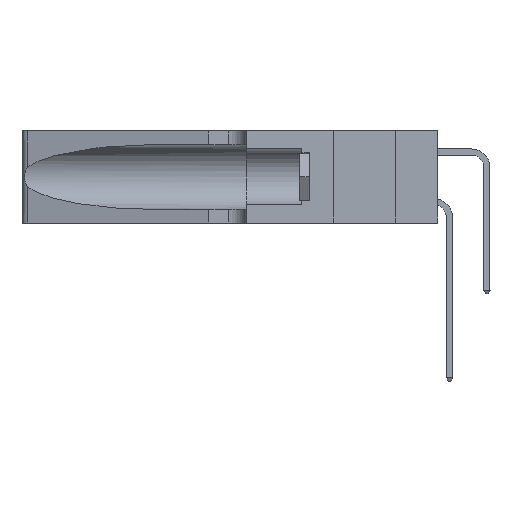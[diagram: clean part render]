
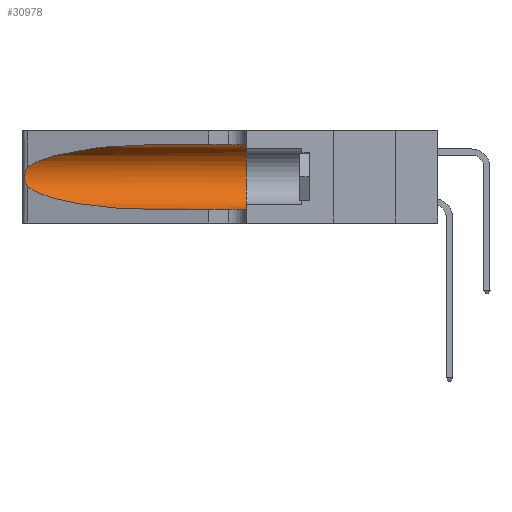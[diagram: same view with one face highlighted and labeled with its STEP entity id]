
A CAD part, left-side view. The second image highlights one B-rep face of the part: STEP entity #30978.
In plain terms, the highlighted cylindrical face has radius 3.308 mm (diameter 6.617 mm), a partial arc.
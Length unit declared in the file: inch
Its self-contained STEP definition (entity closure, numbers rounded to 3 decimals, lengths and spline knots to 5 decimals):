
#34 = CARTESIAN_POINT ( 'NONE',  ( 0.25856, 1.23593, 0.16098 ) ) ;
#484 = CARTESIAN_POINT ( 'NONE',  ( 0.1305, 0.35, 0.185 ) ) ;
#785 = CARTESIAN_POINT ( 'NONE',  ( 0.25487, 1.22718, 0.14631 ) ) ;
#837 = VERTEX_POINT ( 'NONE', #17722 ) ;
#2016 = EDGE_CURVE ( 'NONE', #837, #20874, #7929, .T. ) ;
#2540 = CARTESIAN_POINT ( 'NONE',  ( 0.25487, 1.22718, 0.22369 ) ) ;
#2912 = CARTESIAN_POINT ( 'NONE',  ( 0.25789, 1.23486, 0.15765 ) ) ;
#3282 = CARTESIAN_POINT ( 'NONE',  ( 0.1305, 1.61858, 0.185 ) ) ;
#3753 = CIRCLE ( 'NONE', #21391, 0.13025 ) ;
#3768 = CARTESIAN_POINT ( 'NONE',  ( 0.1305, 0.35, 0.31525 ) ) ;
#4000 = VERTEX_POINT ( 'NONE', #28427 ) ;
#4106 = EDGE_CURVE ( 'NONE', #36669, #4000, #4164, .T. ) ;
#4164 = LINE ( 'NONE', #28540, #14040 ) ;
#5214 = B_SPLINE_CURVE_WITH_KNOTS ( 'NONE', 3,
 ( #2540, #19873, #22757, #31066, #11403, #31175, #34190, #17014, #14859, #34, #2912, #28343, #11272, #25711 ),
 .UNSPECIFIED., .F., .F.,
 ( 4, 2, 2, 2, 2, 2, 4 ),
 ( 0., 0.00027, 0.00053, 0.00107, 0.0016, 0.00187, 0.00214 ),
 .UNSPECIFIED. ) ;
#6984 = VECTOR ( 'NONE', #31416, 39.37008 ) ;
#7235 = EDGE_CURVE ( 'NONE', #20874, #4000, #3753, .T. ) ;
#7929 = LINE ( 'NONE', #8487, #6984 ) ;
#8487 = CARTESIAN_POINT ( 'NONE',  ( 0.1305, 1.61858, 0.31525 ) ) ;
#9735 =( BOUNDED_CURVE ( )  B_SPLINE_CURVE ( 3, ( #10619, #16082, #19103, #21852 ),
 .UNSPECIFIED., .F., .T. ) 
 B_SPLINE_CURVE_WITH_KNOTS ( ( 4, 4 ),
 ( 3.44316, 4.71239 ),
 .UNSPECIFIED. ) 
 CURVE ( )  GEOMETRIC_REPRESENTATION_ITEM ( )  RATIONAL_B_SPLINE_CURVE ( ( 1., 0.87, 0.87, 1. ) ) 
 REPRESENTATION_ITEM ( '' )  );
#10221 = CARTESIAN_POINT ( 'NONE',  ( 0.1305, 0.72297, 0.05475 ) ) ;
#10619 = CARTESIAN_POINT ( 'NONE',  ( 0.25487, 1.22718, 0.14631 ) ) ;
#11245 = EDGE_LOOP ( 'NONE', ( #13324, #26732, #20930, #24260, #18310, #13015 ) ) ;
#11272 = CARTESIAN_POINT ( 'NONE',  ( 0.25555, 1.22993, 0.14849 ) ) ;
#11403 = CARTESIAN_POINT ( 'NONE',  ( 0.25854, 1.2359, 0.20912 ) ) ;
#12745 = EDGE_CURVE ( 'NONE', #21982, #36669, #9735, .T. ) ;
#13015 = ORIENTED_EDGE ( 'NONE', *, *, #2016, .F. ) ;
#13324 = ORIENTED_EDGE ( 'NONE', *, *, #35390, .T. ) ;
#14040 = VECTOR ( 'NONE', #17693, 39.37008 ) ;
#14172 =( BOUNDED_CURVE ( )  B_SPLINE_CURVE ( 3, ( #15383, #24405, #27114, #18531 ),
 .UNSPECIFIED., .F., .F. ) 
 B_SPLINE_CURVE_WITH_KNOTS ( ( 4, 4 ),
 ( 1.5708, 2.84003 ),
 .UNSPECIFIED. ) 
 CURVE ( )  GEOMETRIC_REPRESENTATION_ITEM ( )  RATIONAL_B_SPLINE_CURVE ( ( 1., 0.87, 0.87, 1. ) ) 
 REPRESENTATION_ITEM ( '' )  );
#14859 = CARTESIAN_POINT ( 'NONE',  ( 0.26017, 1.23833, 0.17102 ) ) ;
#15383 = CARTESIAN_POINT ( 'NONE',  ( 0.1305, 0.72297, 0.31525 ) ) ;
#16082 = CARTESIAN_POINT ( 'NONE',  ( 0.2373, 1.15595, 0.08982 ) ) ;
#17014 = CARTESIAN_POINT ( 'NONE',  ( 0.26075, 1.23896, 0.178 ) ) ;
#17378 = DIRECTION ( 'NONE',  ( 0., 0., 1. ) ) ;
#17693 = DIRECTION ( 'NONE',  ( 0., -1., 0. ) ) ;
#17722 = CARTESIAN_POINT ( 'NONE',  ( 0.1305, 0.72297, 0.31525 ) ) ;
#18310 = ORIENTED_EDGE ( 'NONE', *, *, #7235, .F. ) ;
#18531 = CARTESIAN_POINT ( 'NONE',  ( 0.25487, 1.22718, 0.22369 ) ) ;
#19103 = CARTESIAN_POINT ( 'NONE',  ( 0.18966, 0.96281, 0.05475 ) ) ;
#19516 = CYLINDRICAL_SURFACE ( 'NONE', #25426, 0.13025 ) ;
#19873 = CARTESIAN_POINT ( 'NONE',  ( 0.25555, 1.22994, 0.2215 ) ) ;
#20874 = VERTEX_POINT ( 'NONE', #3768 ) ;
#20930 = ORIENTED_EDGE ( 'NONE', *, *, #12745, .T. ) ;
#21391 = AXIS2_PLACEMENT_3D ( 'NONE', #484, #34428, #17378 ) ;
#21852 = CARTESIAN_POINT ( 'NONE',  ( 0.1305, 0.72297, 0.05475 ) ) ;
#21982 = VERTEX_POINT ( 'NONE', #785 ) ;
#22757 = CARTESIAN_POINT ( 'NONE',  ( 0.25639, 1.23184, 0.21858 ) ) ;
#24260 = ORIENTED_EDGE ( 'NONE', *, *, #4106, .T. ) ;
#24405 = CARTESIAN_POINT ( 'NONE',  ( 0.18966, 0.96281, 0.31525 ) ) ;
#24830 = CARTESIAN_POINT ( 'NONE',  ( 0.25487, 1.22718, 0.22369 ) ) ;
#25426 = AXIS2_PLACEMENT_3D ( 'NONE', #3282, #28095, #31812 ) ;
#25711 = CARTESIAN_POINT ( 'NONE',  ( 0.25487, 1.22718, 0.14631 ) ) ;
#26732 = ORIENTED_EDGE ( 'NONE', *, *, #36426, .T. ) ;
#27114 = CARTESIAN_POINT ( 'NONE',  ( 0.2373, 1.15595, 0.28018 ) ) ;
#28095 = DIRECTION ( 'NONE',  ( 0., -1., 0. ) ) ;
#28343 = CARTESIAN_POINT ( 'NONE',  ( 0.25639, 1.23186, 0.15144 ) ) ;
#28427 = CARTESIAN_POINT ( 'NONE',  ( 0.1305, 0.35, 0.05475 ) ) ;
#28540 = CARTESIAN_POINT ( 'NONE',  ( 0.1305, 1.61858, 0.05475 ) ) ;
#29074 = VERTEX_POINT ( 'NONE', #24830 ) ;
#30978 = ADVANCED_FACE ( 'NONE', ( #31956 ), #19516, .F. ) ;
#31066 = CARTESIAN_POINT ( 'NONE',  ( 0.25787, 1.23484, 0.2124 ) ) ;
#31175 = CARTESIAN_POINT ( 'NONE',  ( 0.26018, 1.23835, 0.19895 ) ) ;
#31416 = DIRECTION ( 'NONE',  ( 0., -1., 0. ) ) ;
#31812 = DIRECTION ( 'NONE',  ( 0., 0., -1. ) ) ;
#31956 = FACE_OUTER_BOUND ( 'NONE', #11245, .T. ) ;
#34190 = CARTESIAN_POINT ( 'NONE',  ( 0.26075, 1.23896, 0.19203 ) ) ;
#34428 = DIRECTION ( 'NONE',  ( 0., 1., 0. ) ) ;
#35390 = EDGE_CURVE ( 'NONE', #837, #29074, #14172, .T. ) ;
#36426 = EDGE_CURVE ( 'NONE', #29074, #21982, #5214, .T. ) ;
#36669 = VERTEX_POINT ( 'NONE', #10221 ) ;
